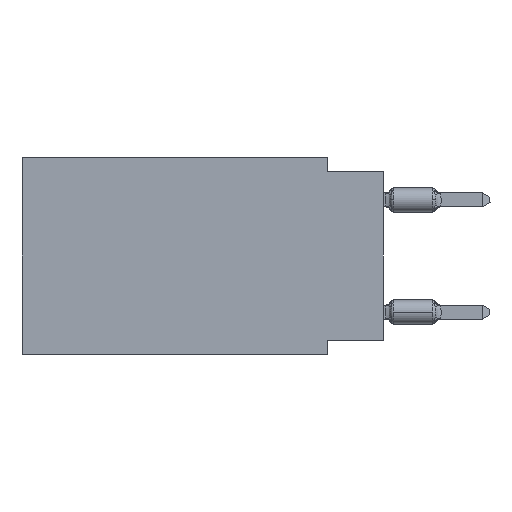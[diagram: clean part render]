
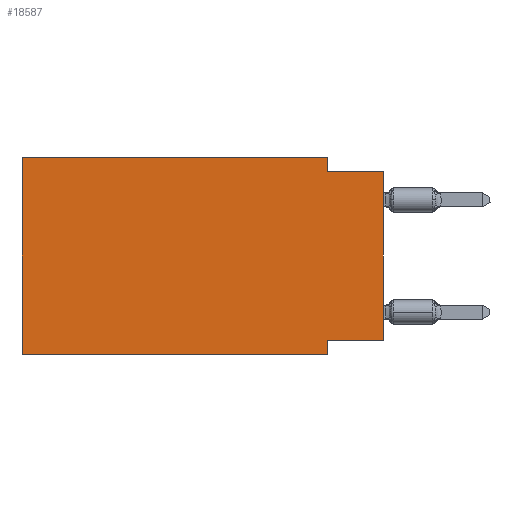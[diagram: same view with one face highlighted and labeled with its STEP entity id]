
A CAD part, left-side view. The second image highlights one B-rep face of the part: STEP entity #18587.
In plain terms, the highlighted planar face has unit normal (-1, 0, 0).
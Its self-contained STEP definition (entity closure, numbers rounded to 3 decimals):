
#112 = VERTEX_POINT ( 'NONE', #20571 ) ;
#788 = VECTOR ( 'NONE', #28063, 1000. ) ;
#889 = LINE ( 'NONE', #18895, #9787 ) ;
#1517 = CARTESIAN_POINT ( 'NONE',  ( 0., 16.383, 0. ) ) ;
#1556 = EDGE_CURVE ( 'NONE', #18121, #112, #12275, .T. ) ;
#1733 = CARTESIAN_POINT ( 'NONE',  ( 0., 0., -0.635 ) ) ;
#2467 = CARTESIAN_POINT ( 'NONE',  ( 0., 16.383, -8.89 ) ) ;
#2610 = LINE ( 'NONE', #2467, #23584 ) ;
#3175 = EDGE_CURVE ( 'NONE', #3259, #21251, #10759, .T. ) ;
#3259 = VERTEX_POINT ( 'NONE', #27270 ) ;
#3906 = DIRECTION ( 'NONE',  ( 0., 0., -1. ) ) ;
#4944 = ORIENTED_EDGE ( 'NONE', *, *, #3175, .F. ) ;
#5603 = LINE ( 'NONE', #14684, #6679 ) ;
#6292 = CARTESIAN_POINT ( 'NONE',  ( 0., 2.54, -8.89 ) ) ;
#6679 = VECTOR ( 'NONE', #23182, 1000. ) ;
#7157 = ORIENTED_EDGE ( 'NONE', *, *, #24958, .T. ) ;
#7508 = VERTEX_POINT ( 'NONE', #11409 ) ;
#7524 = CARTESIAN_POINT ( 'NONE',  ( 0., 16.383, 0. ) ) ;
#7812 = ORIENTED_EDGE ( 'NONE', *, *, #14650, .T. ) ;
#8159 = DIRECTION ( 'NONE',  ( 0., -1., 0. ) ) ;
#9787 = VECTOR ( 'NONE', #19187, 1000. ) ;
#10143 = EDGE_CURVE ( 'NONE', #28857, #18121, #5603, .T. ) ;
#10759 = LINE ( 'NONE', #6292, #13481 ) ;
#10961 = LINE ( 'NONE', #1733, #21759 ) ;
#11409 = CARTESIAN_POINT ( 'NONE',  ( 0., 0., -8.255 ) ) ;
#11700 = CARTESIAN_POINT ( 'NONE',  ( 0., 2.54, -0.635 ) ) ;
#11837 = CARTESIAN_POINT ( 'NONE',  ( 0., 0., -8.255 ) ) ;
#12275 = LINE ( 'NONE', #7524, #21075 ) ;
#13481 = VECTOR ( 'NONE', #17888, 1000. ) ;
#14120 = CARTESIAN_POINT ( 'NONE',  ( 0., 16.383, -8.89 ) ) ;
#14337 = EDGE_CURVE ( 'NONE', #112, #16752, #889, .T. ) ;
#14650 = EDGE_CURVE ( 'NONE', #28857, #21251, #2610, .T. ) ;
#14684 = CARTESIAN_POINT ( 'NONE',  ( 0., 16.383, 0. ) ) ;
#15337 = EDGE_CURVE ( 'NONE', #16752, #28326, #10961, .T. ) ;
#16476 = ORIENTED_EDGE ( 'NONE', *, *, #1556, .F. ) ;
#16692 = ORIENTED_EDGE ( 'NONE', *, *, #14337, .F. ) ;
#16752 = VERTEX_POINT ( 'NONE', #11700 ) ;
#16829 = AXIS2_PLACEMENT_3D ( 'NONE', #1517, #24040, #3906 ) ;
#17447 = FACE_OUTER_BOUND ( 'NONE', #26524, .T. ) ;
#17888 = DIRECTION ( 'NONE',  ( 0., 0., -1. ) ) ;
#18121 = VERTEX_POINT ( 'NONE', #20668 ) ;
#18313 = CARTESIAN_POINT ( 'NONE',  ( 0., 0., -0.635 ) ) ;
#18587 = ADVANCED_FACE ( 'NONE', ( #17447 ), #24321, .F. ) ;
#18895 = CARTESIAN_POINT ( 'NONE',  ( 0., 2.54, 0. ) ) ;
#18965 = ORIENTED_EDGE ( 'NONE', *, *, #15337, .F. ) ;
#18968 = LINE ( 'NONE', #11837, #788 ) ;
#19187 = DIRECTION ( 'NONE',  ( 0., 0., -1. ) ) ;
#20014 = ORIENTED_EDGE ( 'NONE', *, *, #23810, .F. ) ;
#20571 = CARTESIAN_POINT ( 'NONE',  ( 0., 2.54, 0. ) ) ;
#20668 = CARTESIAN_POINT ( 'NONE',  ( 0., 16.383, 0. ) ) ;
#21075 = VECTOR ( 'NONE', #21368, 1000. ) ;
#21251 = VERTEX_POINT ( 'NONE', #28048 ) ;
#21368 = DIRECTION ( 'NONE',  ( 0., -1., 0. ) ) ;
#21759 = VECTOR ( 'NONE', #8159, 1000. ) ;
#22584 = CARTESIAN_POINT ( 'NONE',  ( 0., 0., 0. ) ) ;
#23182 = DIRECTION ( 'NONE',  ( 0., 0., 1. ) ) ;
#23584 = VECTOR ( 'NONE', #24564, 1000. ) ;
#23810 = EDGE_CURVE ( 'NONE', #7508, #3259, #18968, .T. ) ;
#24040 = DIRECTION ( 'NONE',  ( 1., 0., 0. ) ) ;
#24321 = PLANE ( 'NONE',  #16829 ) ;
#24564 = DIRECTION ( 'NONE',  ( 0., -1., 0. ) ) ;
#24820 = LINE ( 'NONE', #22584, #28964 ) ;
#24958 = EDGE_CURVE ( 'NONE', #7508, #28326, #24820, .T. ) ;
#25503 = ORIENTED_EDGE ( 'NONE', *, *, #10143, .F. ) ;
#26524 = EDGE_LOOP ( 'NONE', ( #7157, #18965, #16692, #16476, #25503, #7812, #4944, #20014 ) ) ;
#27270 = CARTESIAN_POINT ( 'NONE',  ( 0., 2.54, -8.255 ) ) ;
#28048 = CARTESIAN_POINT ( 'NONE',  ( 0., 2.54, -8.89 ) ) ;
#28063 = DIRECTION ( 'NONE',  ( 0., 1., 0. ) ) ;
#28326 = VERTEX_POINT ( 'NONE', #18313 ) ;
#28857 = VERTEX_POINT ( 'NONE', #14120 ) ;
#28964 = VECTOR ( 'NONE', #29415, 1000. ) ;
#29415 = DIRECTION ( 'NONE',  ( 0., 0., 1. ) ) ;
